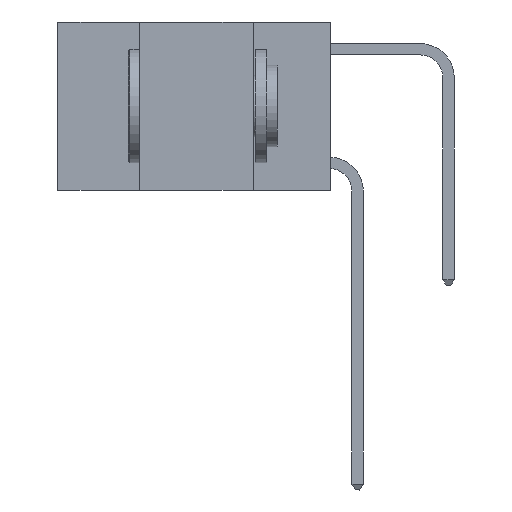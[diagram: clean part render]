
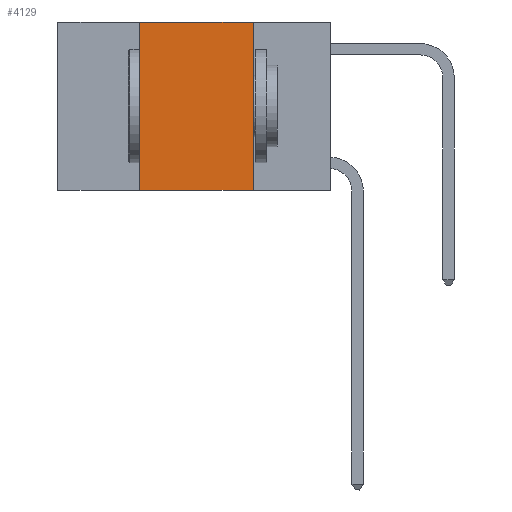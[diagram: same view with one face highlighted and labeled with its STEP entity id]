
A CAD part, left-side view. The second image highlights one B-rep face of the part: STEP entity #4129.
In plain terms, the highlighted planar face has unit normal (-1, 0, 0).
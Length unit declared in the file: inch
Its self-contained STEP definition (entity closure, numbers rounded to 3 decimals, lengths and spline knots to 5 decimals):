
#165 = CARTESIAN_POINT ( 'NONE',  ( 0., 0.42, -0.37 ) ) ;
#497 = ORIENTED_EDGE ( 'NONE', *, *, #8380, .F. ) ;
#569 = DIRECTION ( 'NONE',  ( 0., -1., 0. ) ) ;
#817 = LINE ( 'NONE', #6623, #3264 ) ;
#1023 = DIRECTION ( 'NONE',  ( 0., 0., 1. ) ) ;
#1710 = VECTOR ( 'NONE', #569, 39.37008 ) ;
#2299 = ORIENTED_EDGE ( 'NONE', *, *, #10544, .T. ) ;
#2413 = VERTEX_POINT ( 'NONE', #2582 ) ;
#2477 = ORIENTED_EDGE ( 'NONE', *, *, #10525, .F. ) ;
#2582 = CARTESIAN_POINT ( 'NONE',  ( 0., 0.42, 0. ) ) ;
#3264 = VECTOR ( 'NONE', #1023, 39.37008 ) ;
#3399 = ORIENTED_EDGE ( 'NONE', *, *, #10543, .F. ) ;
#3599 = VECTOR ( 'NONE', #5406, 39.37008 ) ;
#4129 = ADVANCED_FACE ( 'NONE', ( #7648 ), #10803, .F. ) ;
#4168 = VERTEX_POINT ( 'NONE', #10884 ) ;
#5406 = DIRECTION ( 'NONE',  ( 0., 0., -1. ) ) ;
#5698 = DIRECTION ( 'NONE',  ( 0., 0., -1. ) ) ;
#6095 = CARTESIAN_POINT ( 'NONE',  ( 0., 0.6, 0. ) ) ;
#6623 = CARTESIAN_POINT ( 'NONE',  ( 0., 0.42, 0. ) ) ;
#6738 = LINE ( 'NONE', #11566, #3599 ) ;
#7643 = CARTESIAN_POINT ( 'NONE',  ( 0., 0.17, 0. ) ) ;
#7648 = FACE_OUTER_BOUND ( 'NONE', #11386, .T. ) ;
#8028 = VERTEX_POINT ( 'NONE', #165 ) ;
#8380 = EDGE_CURVE ( 'NONE', #2413, #13339, #9885, .T. ) ;
#8839 = CARTESIAN_POINT ( 'NONE',  ( 0., 0.6, 0. ) ) ;
#9885 = LINE ( 'NONE', #6095, #1710 ) ;
#9961 = AXIS2_PLACEMENT_3D ( 'NONE', #8839, #11768, #5698 ) ;
#10525 = EDGE_CURVE ( 'NONE', #13339, #4168, #6738, .T. ) ;
#10543 = EDGE_CURVE ( 'NONE', #8028, #2413, #817, .T. ) ;
#10544 = EDGE_CURVE ( 'NONE', #8028, #4168, #11680, .T. ) ;
#10629 = CARTESIAN_POINT ( 'NONE',  ( 0., 0.6, -0.37 ) ) ;
#10803 = PLANE ( 'NONE',  #9961 ) ;
#10884 = CARTESIAN_POINT ( 'NONE',  ( 0., 0.17, -0.37 ) ) ;
#11381 = VECTOR ( 'NONE', #11603, 39.37008 ) ;
#11386 = EDGE_LOOP ( 'NONE', ( #2477, #497, #3399, #2299 ) ) ;
#11566 = CARTESIAN_POINT ( 'NONE',  ( 0., 0.17, 0. ) ) ;
#11603 = DIRECTION ( 'NONE',  ( 0., -1., 0. ) ) ;
#11680 = LINE ( 'NONE', #10629, #11381 ) ;
#11768 = DIRECTION ( 'NONE',  ( 1., 0., 0. ) ) ;
#13339 = VERTEX_POINT ( 'NONE', #7643 ) ;
